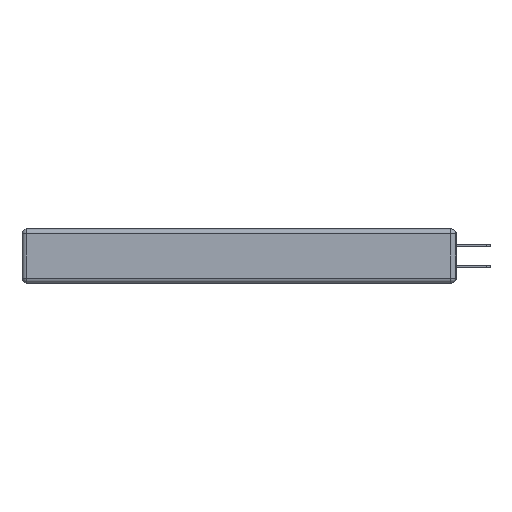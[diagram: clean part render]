
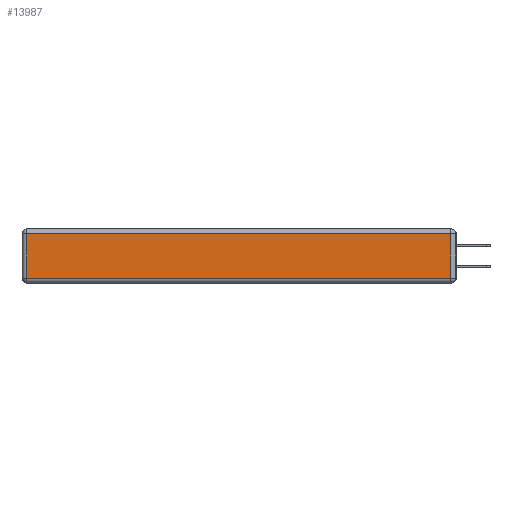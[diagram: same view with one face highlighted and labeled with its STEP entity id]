
A CAD part, left-side view. The second image highlights one B-rep face of the part: STEP entity #13987.
In plain terms, the highlighted planar face has unit normal (-1, 0, 0).
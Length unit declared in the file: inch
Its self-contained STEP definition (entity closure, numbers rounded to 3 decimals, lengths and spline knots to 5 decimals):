
#1024 = ORIENTED_EDGE ( 'NONE', *, *, #7883, .T. ) ;
#1215 = DIRECTION ( 'NONE',  ( 0., 1., 0. ) ) ;
#3135 = CARTESIAN_POINT ( 'NONE',  ( 0., 0.03, -0.313 ) ) ;
#3845 = VERTEX_POINT ( 'NONE', #9401 ) ;
#3982 = VERTEX_POINT ( 'NONE', #7007 ) ;
#4038 = PLANE ( 'NONE',  #15579 ) ;
#4090 = VECTOR ( 'NONE', #1215, 39.37008 ) ;
#4092 = CARTESIAN_POINT ( 'NONE',  ( 0., 2.72, -0.313 ) ) ;
#4174 = EDGE_CURVE ( 'NONE', #3845, #14087, #15896, .T. ) ;
#4407 = VECTOR ( 'NONE', #16198, 39.37008 ) ;
#5120 = ORIENTED_EDGE ( 'NONE', *, *, #4174, .T. ) ;
#5869 = CARTESIAN_POINT ( 'NONE',  ( 0., 0.03, -0.343 ) ) ;
#7007 = CARTESIAN_POINT ( 'NONE',  ( 0., 0.03, -0.03 ) ) ;
#7879 = LINE ( 'NONE', #12467, #10436 ) ;
#7883 = EDGE_CURVE ( 'NONE', #14087, #8271, #7879, .T. ) ;
#7919 = VECTOR ( 'NONE', #9582, 39.37008 ) ;
#7942 = DIRECTION ( 'NONE',  ( 0., 0., 1. ) ) ;
#8271 = VERTEX_POINT ( 'NONE', #3135 ) ;
#8729 = EDGE_LOOP ( 'NONE', ( #1024, #15044, #9050, #5120 ) ) ;
#9050 = ORIENTED_EDGE ( 'NONE', *, *, #14320, .T. ) ;
#9401 = CARTESIAN_POINT ( 'NONE',  ( 0., 2.72, -0.03 ) ) ;
#9582 = DIRECTION ( 'NONE',  ( 0., 0., 1. ) ) ;
#10436 = VECTOR ( 'NONE', #12620, 39.37008 ) ;
#10887 = LINE ( 'NONE', #5869, #7919 ) ;
#11020 = CARTESIAN_POINT ( 'NONE',  ( 0., 2.72, -0.343 ) ) ;
#11217 = CARTESIAN_POINT ( 'NONE',  ( 0., 2.75, -0.03 ) ) ;
#11236 = LINE ( 'NONE', #11217, #4090 ) ;
#11696 = DIRECTION ( 'NONE',  ( -1., 0., 0. ) ) ;
#12467 = CARTESIAN_POINT ( 'NONE',  ( 0., 0., -0.313 ) ) ;
#12620 = DIRECTION ( 'NONE',  ( 0., -1., 0. ) ) ;
#12885 = CARTESIAN_POINT ( 'NONE',  ( 0., 0., -0.343 ) ) ;
#13987 = ADVANCED_FACE ( 'NONE', ( #14189 ), #4038, .T. ) ;
#14087 = VERTEX_POINT ( 'NONE', #4092 ) ;
#14189 = FACE_OUTER_BOUND ( 'NONE', #8729, .T. ) ;
#14320 = EDGE_CURVE ( 'NONE', #3982, #3845, #11236, .T. ) ;
#15044 = ORIENTED_EDGE ( 'NONE', *, *, #16079, .T. ) ;
#15579 = AXIS2_PLACEMENT_3D ( 'NONE', #12885, #11696, #7942 ) ;
#15896 = LINE ( 'NONE', #11020, #4407 ) ;
#16079 = EDGE_CURVE ( 'NONE', #8271, #3982, #10887, .T. ) ;
#16198 = DIRECTION ( 'NONE',  ( 0., 0., -1. ) ) ;
